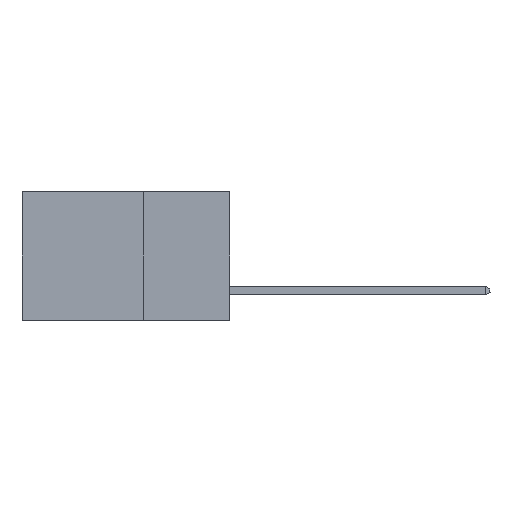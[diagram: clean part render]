
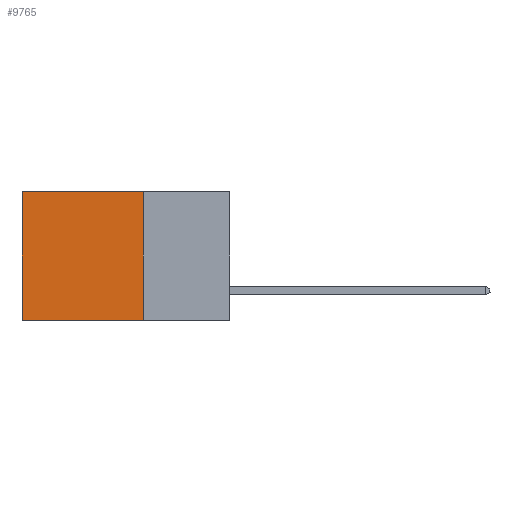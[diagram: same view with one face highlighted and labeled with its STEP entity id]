
A CAD part, left-side view. The second image highlights one B-rep face of the part: STEP entity #9765.
In plain terms, the highlighted planar face has unit normal (-1, 0, 0).
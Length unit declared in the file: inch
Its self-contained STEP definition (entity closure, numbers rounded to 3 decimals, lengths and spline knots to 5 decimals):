
#217 = EDGE_LOOP ( 'NONE', ( #7428, #5651, #8850, #14836 ) ) ;
#348 = CARTESIAN_POINT ( 'NONE',  ( 0.298, 0.25, 0. ) ) ;
#405 = EDGE_CURVE ( 'NONE', #7080, #14155, #7838, .T. ) ;
#1021 = VECTOR ( 'NONE', #5899, 39.37008 ) ;
#1692 = VERTEX_POINT ( 'NONE', #18809 ) ;
#2004 = VECTOR ( 'NONE', #15956, 39.37008 ) ;
#3935 = DIRECTION ( 'NONE',  ( 1., 0., 0. ) ) ;
#4137 = EDGE_CURVE ( 'NONE', #1692, #14155, #20200, .T. ) ;
#4370 = EDGE_CURVE ( 'NONE', #9901, #1692, #7074, .T. ) ;
#5651 = ORIENTED_EDGE ( 'NONE', *, *, #405, .F. ) ;
#5899 = DIRECTION ( 'NONE',  ( 0., 1., 0. ) ) ;
#6809 = AXIS2_PLACEMENT_3D ( 'NONE', #19411, #3935, #14788 ) ;
#7074 = LINE ( 'NONE', #18393, #1021 ) ;
#7080 = VERTEX_POINT ( 'NONE', #18259 ) ;
#7428 = ORIENTED_EDGE ( 'NONE', *, *, #4137, .T. ) ;
#7598 = VECTOR ( 'NONE', #16522, 39.37008 ) ;
#7838 = LINE ( 'NONE', #13598, #7598 ) ;
#8804 = PLANE ( 'NONE',  #6809 ) ;
#8850 = ORIENTED_EDGE ( 'NONE', *, *, #18034, .F. ) ;
#9765 = ADVANCED_FACE ( 'NONE', ( #18275 ), #8804, .F. ) ;
#9901 = VERTEX_POINT ( 'NONE', #348 ) ;
#10696 = VECTOR ( 'NONE', #12970, 39.37008 ) ;
#11208 = CARTESIAN_POINT ( 'NONE',  ( 0.298, 0.25, 0. ) ) ;
#11535 = CARTESIAN_POINT ( 'NONE',  ( 0.298, 0.6, 0. ) ) ;
#12970 = DIRECTION ( 'NONE',  ( 0., 0., -1. ) ) ;
#13598 = CARTESIAN_POINT ( 'NONE',  ( 0.298, 0.25, -0.37 ) ) ;
#14155 = VERTEX_POINT ( 'NONE', #14948 ) ;
#14788 = DIRECTION ( 'NONE',  ( 0., 0., -1. ) ) ;
#14836 = ORIENTED_EDGE ( 'NONE', *, *, #4370, .T. ) ;
#14890 = LINE ( 'NONE', #11208, #2004 ) ;
#14948 = CARTESIAN_POINT ( 'NONE',  ( 0.298, 0.6, -0.37 ) ) ;
#15956 = DIRECTION ( 'NONE',  ( 0., 0., -1. ) ) ;
#16522 = DIRECTION ( 'NONE',  ( 0., 1., 0. ) ) ;
#18034 = EDGE_CURVE ( 'NONE', #9901, #7080, #14890, .T. ) ;
#18259 = CARTESIAN_POINT ( 'NONE',  ( 0.298, 0.25, -0.37 ) ) ;
#18275 = FACE_OUTER_BOUND ( 'NONE', #217, .T. ) ;
#18393 = CARTESIAN_POINT ( 'NONE',  ( 0.298, 0.25, 0. ) ) ;
#18809 = CARTESIAN_POINT ( 'NONE',  ( 0.298, 0.6, 0. ) ) ;
#19411 = CARTESIAN_POINT ( 'NONE',  ( 0.298, 0.25, 0. ) ) ;
#20200 = LINE ( 'NONE', #11535, #10696 ) ;
